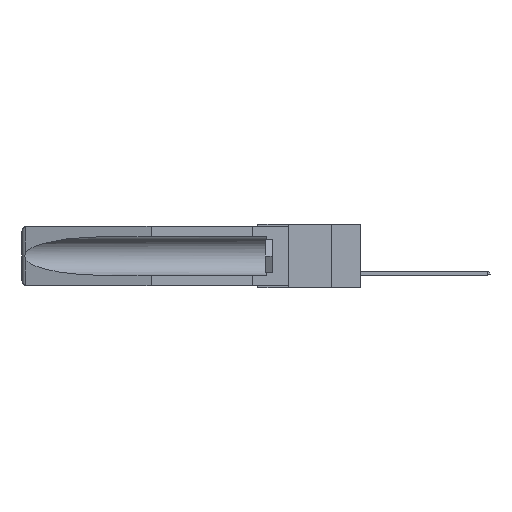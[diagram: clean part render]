
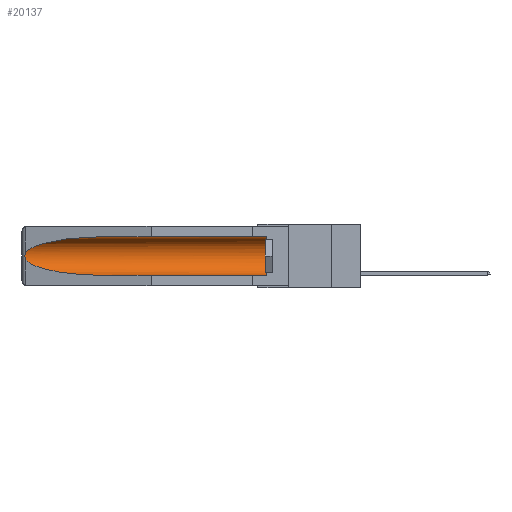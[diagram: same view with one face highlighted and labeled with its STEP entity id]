
A CAD part, left-side view. The second image highlights one B-rep face of the part: STEP entity #20137.
In plain terms, the highlighted cylindrical face has radius 2.857 mm (diameter 5.715 mm), a partial arc.
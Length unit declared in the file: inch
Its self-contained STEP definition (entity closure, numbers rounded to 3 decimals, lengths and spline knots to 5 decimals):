
#69 = CARTESIAN_POINT ( 'NONE',  ( 0.155, 1.07973, -0.059 ) ) ;
#535 = CARTESIAN_POINT ( 'NONE',  ( 0.25451, 1.48313, -0.24835 ) ) ;
#582 = EDGE_CURVE ( 'NONE', #11587, #8056, #10926, .T. ) ;
#1109 =( BOUNDED_CURVE ( )  B_SPLINE_CURVE ( 3, ( #8976, #535, #12898, #19601 ),
 .UNSPECIFIED., .F., .F. ) 
 B_SPLINE_CURVE_WITH_KNOTS ( ( 4, 4 ),
 ( 0.1948, 1.5708 ),
 .UNSPECIFIED. ) 
 CURVE ( )  GEOMETRIC_REPRESENTATION_ITEM ( )  RATIONAL_B_SPLINE_CURVE ( ( 1., 0.848, 0.848, 1. ) ) 
 REPRESENTATION_ITEM ( '' )  );
#1592 = CARTESIAN_POINT ( 'NONE',  ( 0.25451, 1.48313, -0.09465 ) ) ;
#1731 = CARTESIAN_POINT ( 'NONE',  ( 0.26654, 1.53092, -0.15636 ) ) ;
#1808 = CARTESIAN_POINT ( 'NONE',  ( 0.26655, 1.53094, -0.18657 ) ) ;
#2047 =( BOUNDED_CURVE ( )  B_SPLINE_CURVE ( 3, ( #69, #16834, #1592, #13408 ),
 .UNSPECIFIED., .F., .F. ) 
 B_SPLINE_CURVE_WITH_KNOTS ( ( 4, 4 ),
 ( 4.71239, 6.08839 ),
 .UNSPECIFIED. ) 
 CURVE ( )  GEOMETRIC_REPRESENTATION_ITEM ( )  RATIONAL_B_SPLINE_CURVE ( ( 1., 0.848, 0.848, 1. ) ) 
 REPRESENTATION_ITEM ( '' )  );
#2537 = EDGE_CURVE ( 'NONE', #18428, #11569, #17892, .T. ) ;
#2837 = ORIENTED_EDGE ( 'NONE', *, *, #14373, .T. ) ;
#3467 = DIRECTION ( 'NONE',  ( 0., -1., 0. ) ) ;
#4953 = CARTESIAN_POINT ( 'NONE',  ( 0.155, 0.126, -0.1715 ) ) ;
#5334 = CARTESIAN_POINT ( 'NONE',  ( 0.26537, 1.52718, -0.14972 ) ) ;
#5384 = FACE_OUTER_BOUND ( 'NONE', #17296, .T. ) ;
#6200 = VECTOR ( 'NONE', #12556, 39.37008 ) ;
#6324 = VERTEX_POINT ( 'NONE', #14258 ) ;
#6358 = EDGE_CURVE ( 'NONE', #11569, #12837, #1109, .T. ) ;
#6572 = DIRECTION ( 'NONE',  ( 0., 1., 0. ) ) ;
#6779 = CARTESIAN_POINT ( 'NONE',  ( 0.26597, 1.52961, -0.15275 ) ) ;
#6877 = DIRECTION ( 'NONE',  ( 0., 0., 1. ) ) ;
#7027 = ORIENTED_EDGE ( 'NONE', *, *, #582, .T. ) ;
#7420 = AXIS2_PLACEMENT_3D ( 'NONE', #20031, #21736, #19804 ) ;
#8056 = VERTEX_POINT ( 'NONE', #12020 ) ;
#8485 = CARTESIAN_POINT ( 'NONE',  ( 0.2675, 1.53308, -0.16763 ) ) ;
#8592 = VECTOR ( 'NONE', #6572, 39.37008 ) ;
#8976 = CARTESIAN_POINT ( 'NONE',  ( 0.26537, 1.52718, -0.19328 ) ) ;
#9153 = CARTESIAN_POINT ( 'NONE',  ( 0.155, -0.30754, -0.059 ) ) ;
#9370 = CARTESIAN_POINT ( 'NONE',  ( 0.155, 1.07973, -0.284 ) ) ;
#9847 = ORIENTED_EDGE ( 'NONE', *, *, #19743, .T. ) ;
#10197 = CARTESIAN_POINT ( 'NONE',  ( 0.26537, 1.52718, -0.19328 ) ) ;
#10339 = CARTESIAN_POINT ( 'NONE',  ( 0.2673, 1.53269, -0.17917 ) ) ;
#10700 = ORIENTED_EDGE ( 'NONE', *, *, #2537, .T. ) ;
#10926 = CIRCLE ( 'NONE', #21755, 0.1125 ) ;
#11569 = VERTEX_POINT ( 'NONE', #18769 ) ;
#11587 = VERTEX_POINT ( 'NONE', #18199 ) ;
#12020 = CARTESIAN_POINT ( 'NONE',  ( 0.155, 0.126, -0.059 ) ) ;
#12401 = ORIENTED_EDGE ( 'NONE', *, *, #6358, .T. ) ;
#12556 = DIRECTION ( 'NONE',  ( 0., 1., 0. ) ) ;
#12837 = VERTEX_POINT ( 'NONE', #9370 ) ;
#12898 = CARTESIAN_POINT ( 'NONE',  ( 0.21114, 1.30732, -0.284 ) ) ;
#13109 = LINE ( 'NONE', #13501, #8592 ) ;
#13371 = CYLINDRICAL_SURFACE ( 'NONE', #7420, 0.1125 ) ;
#13408 = CARTESIAN_POINT ( 'NONE',  ( 0.26537, 1.52718, -0.14972 ) ) ;
#13501 = CARTESIAN_POINT ( 'NONE',  ( 0.155, -0.30754, -0.284 ) ) ;
#14076 = ORIENTED_EDGE ( 'NONE', *, *, #19337, .F. ) ;
#14258 = CARTESIAN_POINT ( 'NONE',  ( 0.155, 1.07973, -0.059 ) ) ;
#14373 = EDGE_CURVE ( 'NONE', #6324, #18428, #2047, .T. ) ;
#15328 = CARTESIAN_POINT ( 'NONE',  ( 0.26597, 1.5296, -0.19026 ) ) ;
#16834 = CARTESIAN_POINT ( 'NONE',  ( 0.21114, 1.30732, -0.059 ) ) ;
#16977 = CARTESIAN_POINT ( 'NONE',  ( 0.26537, 1.52718, -0.14972 ) ) ;
#17296 = EDGE_LOOP ( 'NONE', ( #2837, #10700, #12401, #14076, #7027, #9847 ) ) ;
#17892 = B_SPLINE_CURVE_WITH_KNOTS ( 'NONE', 3,
 ( #16977, #6779, #1731, #18870, #8485, #20364, #10339, #1808, #15328, #10197 ),
 .UNSPECIFIED., .F., .F.,
 ( 4, 2, 2, 2, 4 ),
 ( 0., 0.00029, 0.00058, 0.00087, 0.00117 ),
 .UNSPECIFIED. ) ;
#18199 = CARTESIAN_POINT ( 'NONE',  ( 0.155, 0.126, -0.284 ) ) ;
#18428 = VERTEX_POINT ( 'NONE', #5334 ) ;
#18438 = LINE ( 'NONE', #9153, #6200 ) ;
#18769 = CARTESIAN_POINT ( 'NONE',  ( 0.26537, 1.52718, -0.19328 ) ) ;
#18870 = CARTESIAN_POINT ( 'NONE',  ( 0.2673, 1.5327, -0.16383 ) ) ;
#19337 = EDGE_CURVE ( 'NONE', #11587, #12837, #13109, .T. ) ;
#19601 = CARTESIAN_POINT ( 'NONE',  ( 0.155, 1.07973, -0.284 ) ) ;
#19743 = EDGE_CURVE ( 'NONE', #8056, #6324, #18438, .T. ) ;
#19804 = DIRECTION ( 'NONE',  ( 0., 0., 1. ) ) ;
#20031 = CARTESIAN_POINT ( 'NONE',  ( 0.155, -0.30754, -0.1715 ) ) ;
#20137 = ADVANCED_FACE ( 'NONE', ( #5384 ), #13371, .F. ) ;
#20364 = CARTESIAN_POINT ( 'NONE',  ( 0.2675, 1.53308, -0.17534 ) ) ;
#21736 = DIRECTION ( 'NONE',  ( 0., 1., 0. ) ) ;
#21755 = AXIS2_PLACEMENT_3D ( 'NONE', #4953, #3467, #6877 ) ;
